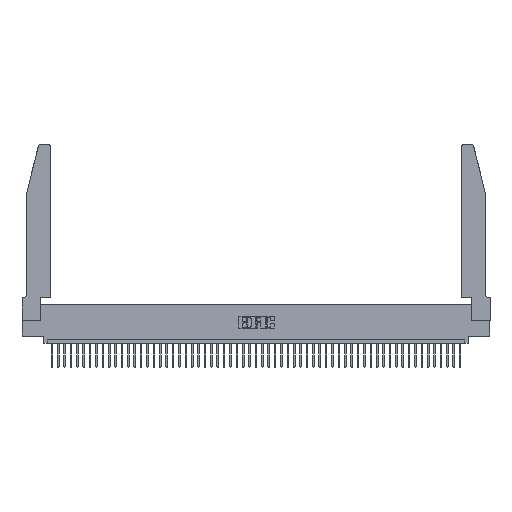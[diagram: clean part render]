
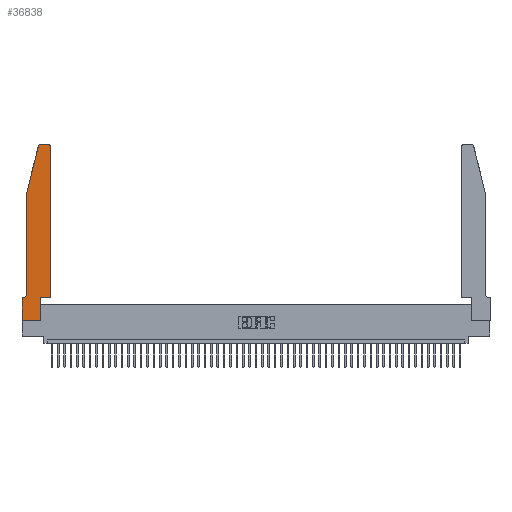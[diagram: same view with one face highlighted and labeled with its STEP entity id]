
A CAD part, top view. The second image highlights one B-rep face of the part: STEP entity #36838.
In plain terms, the highlighted planar face has unit normal (0, 0, 1).
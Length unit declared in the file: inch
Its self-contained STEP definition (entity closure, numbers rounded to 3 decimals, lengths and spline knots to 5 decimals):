
#1180 = CARTESIAN_POINT ( 'NONE',  ( 0., 0.35, 0.37 ) ) ;
#1479 = LINE ( 'NONE', #47416, #43696 ) ;
#1988 = DIRECTION ( 'NONE',  ( -1., 0., 0. ) ) ;
#2232 = VERTEX_POINT ( 'NONE', #11102 ) ;
#2268 = DIRECTION ( 'NONE',  ( -1., 0., 0. ) ) ;
#3376 = AXIS2_PLACEMENT_3D ( 'NONE', #15673, #7692, #19616 ) ;
#4043 = CIRCLE ( 'NONE', #27728, 0.03 ) ;
#4349 = ORIENTED_EDGE ( 'NONE', *, *, #32454, .T. ) ;
#4891 = ORIENTED_EDGE ( 'NONE', *, *, #32842, .T. ) ;
#5456 = CIRCLE ( 'NONE', #48368, 0.07 ) ;
#6065 = CARTESIAN_POINT ( 'NONE',  ( 0.2865, 0., 0.37 ) ) ;
#6199 = EDGE_CURVE ( 'NONE', #11430, #16672, #25350, .T. ) ;
#6257 = LINE ( 'NONE', #37079, #28249 ) ;
#7168 = DIRECTION ( 'NONE',  ( 0., -1., 0. ) ) ;
#7177 = CARTESIAN_POINT ( 'NONE',  ( 0.0755, 2., 0.37 ) ) ;
#7692 = DIRECTION ( 'NONE',  ( 0., 0., 1. ) ) ;
#8345 = VECTOR ( 'NONE', #11049, 39.37008 ) ;
#8813 = FACE_OUTER_BOUND ( 'NONE', #47952, .T. ) ;
#8874 = LINE ( 'NONE', #47544, #29048 ) ;
#9797 = CARTESIAN_POINT ( 'NONE',  ( 0.0055, 0.35, 0.37 ) ) ;
#10914 = EDGE_CURVE ( 'NONE', #34900, #31813, #20549, .T. ) ;
#11049 = DIRECTION ( 'NONE',  ( 1., 0., 0. ) ) ;
#11102 = CARTESIAN_POINT ( 'NONE',  ( 0.0755, 0.42, 0.37 ) ) ;
#11384 = CARTESIAN_POINT ( 'NONE',  ( 0.4205, 2.72, 0.37 ) ) ;
#11430 = VERTEX_POINT ( 'NONE', #9797 ) ;
#11669 = AXIS2_PLACEMENT_3D ( 'NONE', #11384, #22720, #31053 ) ;
#12510 = ORIENTED_EDGE ( 'NONE', *, *, #10914, .T. ) ;
#12652 = VERTEX_POINT ( 'NONE', #7177 ) ;
#12729 = VERTEX_POINT ( 'NONE', #31364 ) ;
#13821 = ORIENTED_EDGE ( 'NONE', *, *, #42365, .T. ) ;
#14139 = CIRCLE ( 'NONE', #11669, 0.03 ) ;
#14864 = ORIENTED_EDGE ( 'NONE', *, *, #22188, .T. ) ;
#15673 = CARTESIAN_POINT ( 'NONE',  ( 0., 0.35, 0.37 ) ) ;
#16672 = VERTEX_POINT ( 'NONE', #1180 ) ;
#16776 = EDGE_CURVE ( 'NONE', #12652, #2232, #6257, .T. ) ;
#19616 = DIRECTION ( 'NONE',  ( 1., 0., 0. ) ) ;
#20321 = VECTOR ( 'NONE', #50095, 39.37008 ) ;
#20472 = CARTESIAN_POINT ( 'NONE',  ( 0.284, 2.75, 0.37 ) ) ;
#20549 = LINE ( 'NONE', #50634, #8345 ) ;
#20590 = CARTESIAN_POINT ( 'NONE',  ( 0.284, 2.72, 0.37 ) ) ;
#20958 = DIRECTION ( 'NONE',  ( 0., 0., 1. ) ) ;
#21178 = EDGE_CURVE ( 'NONE', #23800, #40435, #8874, .T. ) ;
#21520 = ORIENTED_EDGE ( 'NONE', *, *, #6199, .T. ) ;
#21750 = EDGE_CURVE ( 'NONE', #31813, #41060, #31425, .T. ) ;
#22188 = EDGE_CURVE ( 'NONE', #12729, #12652, #41228, .T. ) ;
#22720 = DIRECTION ( 'NONE',  ( 0., 0., 1. ) ) ;
#23233 = PLANE ( 'NONE',  #3376 ) ;
#23573 = ORIENTED_EDGE ( 'NONE', *, *, #44168, .T. ) ;
#23800 = VERTEX_POINT ( 'NONE', #31396 ) ;
#24759 = CARTESIAN_POINT ( 'NONE',  ( 0.4505, 2.72, 0.37 ) ) ;
#25218 = LINE ( 'NONE', #38842, #39934 ) ;
#25347 = CARTESIAN_POINT ( 'NONE',  ( 0.0055, 0.42, 0.37 ) ) ;
#25350 = LINE ( 'NONE', #49000, #47450 ) ;
#26742 = CARTESIAN_POINT ( 'NONE',  ( 0.0755, 2., 0.37 ) ) ;
#26828 = VERTEX_POINT ( 'NONE', #49737 ) ;
#26994 = ORIENTED_EDGE ( 'NONE', *, *, #16776, .T. ) ;
#27327 = CARTESIAN_POINT ( 'NONE',  ( 0.2605, 2.75, 0.37 ) ) ;
#27728 = AXIS2_PLACEMENT_3D ( 'NONE', #20590, #20958, #40321 ) ;
#28201 = EDGE_CURVE ( 'NONE', #2232, #11430, #5456, .T. ) ;
#28249 = VECTOR ( 'NONE', #29679, 39.37008 ) ;
#28983 = DIRECTION ( 'NONE',  ( 0., 1., 0. ) ) ;
#29048 = VECTOR ( 'NONE', #35844, 39.37008 ) ;
#29679 = DIRECTION ( 'NONE',  ( 0., -1., 0. ) ) ;
#29940 = ORIENTED_EDGE ( 'NONE', *, *, #28201, .T. ) ;
#30974 = VECTOR ( 'NONE', #31260, 39.37008 ) ;
#31053 = DIRECTION ( 'NONE',  ( 1., 0., 0. ) ) ;
#31260 = DIRECTION ( 'NONE',  ( -1., 0., 0. ) ) ;
#31364 = CARTESIAN_POINT ( 'NONE',  ( 0.25487, 2.72718, 0.37 ) ) ;
#31396 = CARTESIAN_POINT ( 'NONE',  ( 0.4505, 0.35, 0.37 ) ) ;
#31425 = LINE ( 'NONE', #36735, #39428 ) ;
#31813 = VERTEX_POINT ( 'NONE', #6065 ) ;
#32128 = DIRECTION ( 'NONE',  ( 1., 0., 0. ) ) ;
#32454 = EDGE_CURVE ( 'NONE', #16672, #34900, #25218, .T. ) ;
#32842 = EDGE_CURVE ( 'NONE', #40435, #26828, #14139, .T. ) ;
#33501 = LINE ( 'NONE', #27327, #30974 ) ;
#34900 = VERTEX_POINT ( 'NONE', #38008 ) ;
#35844 = DIRECTION ( 'NONE',  ( 0., 1., 0. ) ) ;
#36735 = CARTESIAN_POINT ( 'NONE',  ( 0.2865, 0.35, 0.37 ) ) ;
#36838 = ADVANCED_FACE ( 'NONE', ( #8813 ), #23233, .T. ) ;
#37079 = CARTESIAN_POINT ( 'NONE',  ( 0.0755, 2., 0.37 ) ) ;
#38008 = CARTESIAN_POINT ( 'NONE',  ( 0., 0., 0.37 ) ) ;
#38084 = ORIENTED_EDGE ( 'NONE', *, *, #21750, .T. ) ;
#38842 = CARTESIAN_POINT ( 'NONE',  ( 0., 0., 0.37 ) ) ;
#39042 = VERTEX_POINT ( 'NONE', #20472 ) ;
#39428 = VECTOR ( 'NONE', #28983, 39.37008 ) ;
#39934 = VECTOR ( 'NONE', #7168, 39.37008 ) ;
#40321 = DIRECTION ( 'NONE',  ( 1., 0., 0. ) ) ;
#40435 = VERTEX_POINT ( 'NONE', #24759 ) ;
#40791 = DIRECTION ( 'NONE',  ( 0., 0., -1. ) ) ;
#41060 = VERTEX_POINT ( 'NONE', #44294 ) ;
#41228 = LINE ( 'NONE', #26742, #20321 ) ;
#42365 = EDGE_CURVE ( 'NONE', #26828, #39042, #33501, .T. ) ;
#42953 = EDGE_CURVE ( 'NONE', #39042, #12729, #4043, .T. ) ;
#43696 = VECTOR ( 'NONE', #32128, 39.37008 ) ;
#44168 = EDGE_CURVE ( 'NONE', #41060, #23800, #1479, .T. ) ;
#44294 = CARTESIAN_POINT ( 'NONE',  ( 0.2865, 0.35, 0.37 ) ) ;
#47416 = CARTESIAN_POINT ( 'NONE',  ( 0.4505, 0.35, 0.37 ) ) ;
#47450 = VECTOR ( 'NONE', #2268, 39.37008 ) ;
#47544 = CARTESIAN_POINT ( 'NONE',  ( 0.4505, 0.35, 0.37 ) ) ;
#47613 = ORIENTED_EDGE ( 'NONE', *, *, #21178, .T. ) ;
#47952 = EDGE_LOOP ( 'NONE', ( #13821, #48620, #14864, #26994, #29940, #21520, #4349, #12510, #38084, #23573, #47613, #4891 ) ) ;
#48368 = AXIS2_PLACEMENT_3D ( 'NONE', #25347, #40791, #1988 ) ;
#48620 = ORIENTED_EDGE ( 'NONE', *, *, #42953, .T. ) ;
#49000 = CARTESIAN_POINT ( 'NONE',  ( 0.0755, 0.35, 0.37 ) ) ;
#49737 = CARTESIAN_POINT ( 'NONE',  ( 0.4205, 2.75, 0.37 ) ) ;
#50095 = DIRECTION ( 'NONE',  ( -0.239, -0.971, 0. ) ) ;
#50634 = CARTESIAN_POINT ( 'NONE',  ( 0., 0., 0.37 ) ) ;
